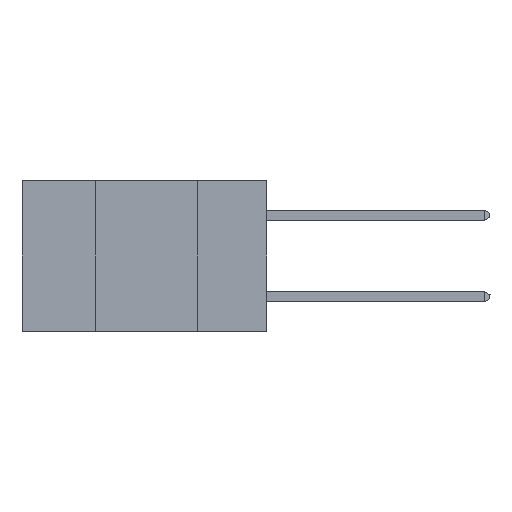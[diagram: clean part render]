
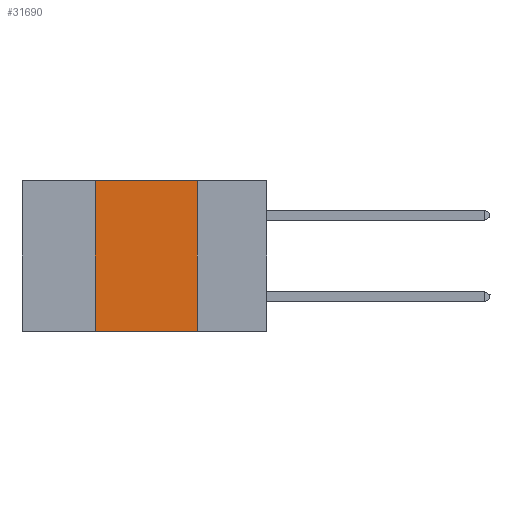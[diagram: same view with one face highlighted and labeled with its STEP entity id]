
A CAD part, left-side view. The second image highlights one B-rep face of the part: STEP entity #31690.
In plain terms, the highlighted planar face has unit normal (-1, 0, 0).
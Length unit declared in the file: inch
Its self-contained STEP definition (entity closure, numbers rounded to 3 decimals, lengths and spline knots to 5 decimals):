
#862 = LINE ( 'NONE', #35497, #20107 ) ;
#1438 = CARTESIAN_POINT ( 'NONE',  ( 0., 0.6, 0. ) ) ;
#3082 = ORIENTED_EDGE ( 'NONE', *, *, #9671, .F. ) ;
#3387 = EDGE_LOOP ( 'NONE', ( #15174, #36636, #3082, #39829 ) ) ;
#6487 = CARTESIAN_POINT ( 'NONE',  ( 0., 0.42, 0. ) ) ;
#6515 = AXIS2_PLACEMENT_3D ( 'NONE', #22701, #23122, #10133 ) ;
#7607 = LINE ( 'NONE', #29050, #37252 ) ;
#8568 = CARTESIAN_POINT ( 'NONE',  ( 0., 0.42, 0. ) ) ;
#9671 = EDGE_CURVE ( 'NONE', #26985, #35115, #28330, .T. ) ;
#10133 = DIRECTION ( 'NONE',  ( 0., 0., -1. ) ) ;
#13036 = FACE_OUTER_BOUND ( 'NONE', #3387, .T. ) ;
#13540 = CARTESIAN_POINT ( 'NONE',  ( 0., 0.42, -0.37 ) ) ;
#13959 = VERTEX_POINT ( 'NONE', #26065 ) ;
#13992 = DIRECTION ( 'NONE',  ( 0., -1., 0. ) ) ;
#15174 = ORIENTED_EDGE ( 'NONE', *, *, #37087, .F. ) ;
#16666 = DIRECTION ( 'NONE',  ( 0., -1., 0. ) ) ;
#20107 = VECTOR ( 'NONE', #29906, 39.37008 ) ;
#20171 = CARTESIAN_POINT ( 'NONE',  ( 0., 0.17, -0.37 ) ) ;
#22701 = CARTESIAN_POINT ( 'NONE',  ( 0., 0.6, 0. ) ) ;
#22741 = DIRECTION ( 'NONE',  ( 0., 0., 1. ) ) ;
#23122 = DIRECTION ( 'NONE',  ( 1., 0., 0. ) ) ;
#26065 = CARTESIAN_POINT ( 'NONE',  ( 0., 0.17, 0. ) ) ;
#26592 = EDGE_CURVE ( 'NONE', #26985, #39279, #7607, .T. ) ;
#26985 = VERTEX_POINT ( 'NONE', #13540 ) ;
#28330 = LINE ( 'NONE', #6487, #29896 ) ;
#28667 = VECTOR ( 'NONE', #16666, 39.37008 ) ;
#29050 = CARTESIAN_POINT ( 'NONE',  ( 0., 0.6, -0.37 ) ) ;
#29896 = VECTOR ( 'NONE', #22741, 39.37008 ) ;
#29906 = DIRECTION ( 'NONE',  ( 0., 0., -1. ) ) ;
#31690 = ADVANCED_FACE ( 'NONE', ( #13036 ), #38576, .F. ) ;
#35115 = VERTEX_POINT ( 'NONE', #8568 ) ;
#35451 = LINE ( 'NONE', #1438, #28667 ) ;
#35497 = CARTESIAN_POINT ( 'NONE',  ( 0., 0.17, 0. ) ) ;
#36636 = ORIENTED_EDGE ( 'NONE', *, *, #37552, .F. ) ;
#37087 = EDGE_CURVE ( 'NONE', #13959, #39279, #862, .T. ) ;
#37252 = VECTOR ( 'NONE', #13992, 39.37008 ) ;
#37552 = EDGE_CURVE ( 'NONE', #35115, #13959, #35451, .T. ) ;
#38576 = PLANE ( 'NONE',  #6515 ) ;
#39279 = VERTEX_POINT ( 'NONE', #20171 ) ;
#39829 = ORIENTED_EDGE ( 'NONE', *, *, #26592, .T. ) ;
